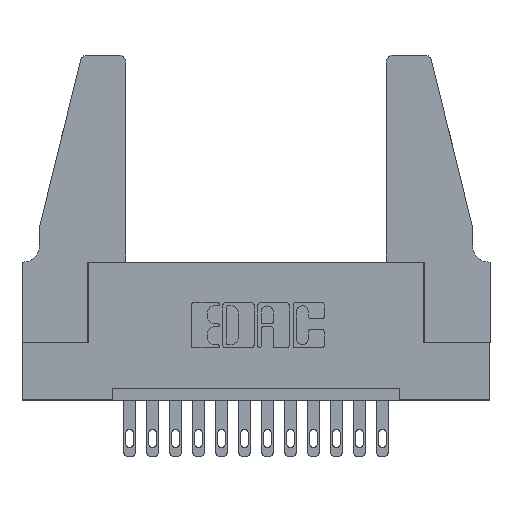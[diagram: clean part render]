
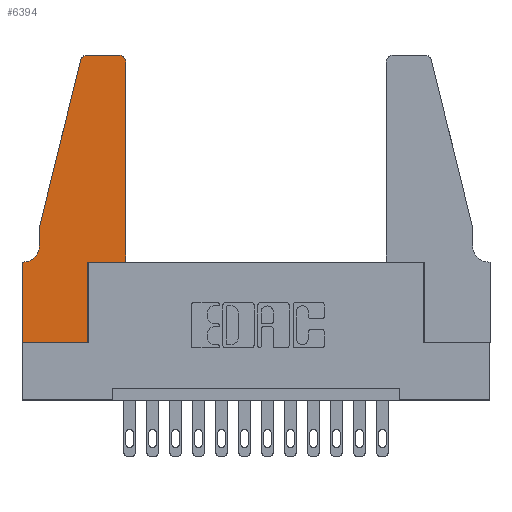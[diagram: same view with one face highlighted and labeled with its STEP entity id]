
A CAD part, top view. The second image highlights one B-rep face of the part: STEP entity #6394.
In plain terms, the highlighted planar face has unit normal (0, 0, 1).
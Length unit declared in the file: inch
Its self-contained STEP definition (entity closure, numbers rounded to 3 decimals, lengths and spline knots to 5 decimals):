
#30 = VERTEX_POINT ( 'NONE', #172 ) ;
#31 = CARTESIAN_POINT ( 'NONE',  ( 0.4505, 0.35, 0.37 ) ) ;
#32 = AXIS2_PLACEMENT_3D ( 'NONE', #9577, #11990, #8432 ) ;
#115 = CARTESIAN_POINT ( 'NONE',  ( 0.25487, 1.22718, 0.37 ) ) ;
#172 = CARTESIAN_POINT ( 'NONE',  ( 0.2865, 0.35, 0.37 ) ) ;
#289 = ORIENTED_EDGE ( 'NONE', *, *, #7589, .T. ) ;
#372 = ORIENTED_EDGE ( 'NONE', *, *, #15129, .T. ) ;
#528 = VECTOR ( 'NONE', #3207, 39.37008 ) ;
#712 = EDGE_CURVE ( 'NONE', #8361, #4221, #1528, .T. ) ;
#730 = CARTESIAN_POINT ( 'NONE',  ( 0.0055, 0.42, 0.37 ) ) ;
#919 = ORIENTED_EDGE ( 'NONE', *, *, #4706, .T. ) ;
#1107 = AXIS2_PLACEMENT_3D ( 'NONE', #2877, #8694, #6245 ) ;
#1387 = EDGE_CURVE ( 'NONE', #13014, #14418, #3705, .T. ) ;
#1528 = LINE ( 'NONE', #14785, #4673 ) ;
#1633 = EDGE_CURVE ( 'NONE', #4221, #30, #10145, .T. ) ;
#1637 = CARTESIAN_POINT ( 'NONE',  ( 0.4505, 1.22, 0.37 ) ) ;
#1676 = VECTOR ( 'NONE', #13841, 39.37008 ) ;
#1745 = CARTESIAN_POINT ( 'NONE',  ( 0., 0.35, 0.37 ) ) ;
#1811 = DIRECTION ( 'NONE',  ( 0., 0., 1. ) ) ;
#2015 = CARTESIAN_POINT ( 'NONE',  ( 0.0755, 0.5, 0.37 ) ) ;
#2060 = CARTESIAN_POINT ( 'NONE',  ( 0.284, 1.25, 0.37 ) ) ;
#2197 = LINE ( 'NONE', #2015, #528 ) ;
#2347 = LINE ( 'NONE', #13626, #3091 ) ;
#2384 = VERTEX_POINT ( 'NONE', #12942 ) ;
#2505 = DIRECTION ( 'NONE',  ( 1., 0., 0. ) ) ;
#2577 = CARTESIAN_POINT ( 'NONE',  ( 0.4505, 0.35, 0.37 ) ) ;
#2704 = LINE ( 'NONE', #10764, #11708 ) ;
#2785 = CIRCLE ( 'NONE', #12614, 0.07 ) ;
#2877 = CARTESIAN_POINT ( 'NONE',  ( 0.4205, 1.22, 0.37 ) ) ;
#3021 = DIRECTION ( 'NONE',  ( 1., 0., 0. ) ) ;
#3059 = PLANE ( 'NONE',  #10366 ) ;
#3091 = VECTOR ( 'NONE', #6474, 39.37008 ) ;
#3207 = DIRECTION ( 'NONE',  ( 0., -1., 0. ) ) ;
#3345 = EDGE_CURVE ( 'NONE', #12278, #14590, #2347, .T. ) ;
#3368 = VECTOR ( 'NONE', #6149, 39.37008 ) ;
#3610 = ORIENTED_EDGE ( 'NONE', *, *, #10073, .T. ) ;
#3705 = LINE ( 'NONE', #11720, #1676 ) ;
#4221 = VERTEX_POINT ( 'NONE', #15079 ) ;
#4346 = VERTEX_POINT ( 'NONE', #115 ) ;
#4609 = LINE ( 'NONE', #13821, #6424 ) ;
#4642 = CIRCLE ( 'NONE', #32, 0.03 ) ;
#4673 = VECTOR ( 'NONE', #6603, 39.37008 ) ;
#4704 = CIRCLE ( 'NONE', #1107, 0.03 ) ;
#4706 = EDGE_CURVE ( 'NONE', #14180, #12278, #4704, .T. ) ;
#5219 = ORIENTED_EDGE ( 'NONE', *, *, #13442, .T. ) ;
#5308 = ORIENTED_EDGE ( 'NONE', *, *, #712, .T. ) ;
#5489 = DIRECTION ( 'NONE',  ( -0.239, -0.971, 0. ) ) ;
#6100 = CARTESIAN_POINT ( 'NONE',  ( 0.2865, 0.35, 0.37 ) ) ;
#6149 = DIRECTION ( 'NONE',  ( 0., 1., 0. ) ) ;
#6245 = DIRECTION ( 'NONE',  ( 1., 0., 0. ) ) ;
#6394 = ADVANCED_FACE ( 'NONE', ( #14870 ), #3059, .T. ) ;
#6424 = VECTOR ( 'NONE', #5489, 39.37008 ) ;
#6474 = DIRECTION ( 'NONE',  ( -1., 0., 0. ) ) ;
#6603 = DIRECTION ( 'NONE',  ( 1., 0., 0. ) ) ;
#6948 = ORIENTED_EDGE ( 'NONE', *, *, #1387, .T. ) ;
#7041 = DIRECTION ( 'NONE',  ( 0., -1., 0. ) ) ;
#7384 = EDGE_CURVE ( 'NONE', #14590, #4346, #4642, .T. ) ;
#7427 = CARTESIAN_POINT ( 'NONE',  ( 0.4205, 1.25, 0.37 ) ) ;
#7589 = EDGE_CURVE ( 'NONE', #2384, #13014, #2785, .T. ) ;
#7730 = VECTOR ( 'NONE', #9360, 39.37008 ) ;
#8361 = VERTEX_POINT ( 'NONE', #8669 ) ;
#8432 = DIRECTION ( 'NONE',  ( 1., 0., 0. ) ) ;
#8627 = LINE ( 'NONE', #9400, #13401 ) ;
#8669 = CARTESIAN_POINT ( 'NONE',  ( 0., 0., 0.37 ) ) ;
#8694 = DIRECTION ( 'NONE',  ( 0., 0., 1. ) ) ;
#9360 = DIRECTION ( 'NONE',  ( 0., 1., 0. ) ) ;
#9400 = CARTESIAN_POINT ( 'NONE',  ( 0., 0., 0.37 ) ) ;
#9577 = CARTESIAN_POINT ( 'NONE',  ( 0.284, 1.22, 0.37 ) ) ;
#9772 = CARTESIAN_POINT ( 'NONE',  ( 0.0755, 0.5, 0.37 ) ) ;
#10073 = EDGE_CURVE ( 'NONE', #12759, #2384, #2197, .T. ) ;
#10145 = LINE ( 'NONE', #6100, #3368 ) ;
#10175 = ORIENTED_EDGE ( 'NONE', *, *, #11616, .T. ) ;
#10305 = ORIENTED_EDGE ( 'NONE', *, *, #7384, .T. ) ;
#10366 = AXIS2_PLACEMENT_3D ( 'NONE', #11344, #1811, #3021 ) ;
#10739 = CARTESIAN_POINT ( 'NONE',  ( 0.0055, 0.35, 0.37 ) ) ;
#10764 = CARTESIAN_POINT ( 'NONE',  ( 0.4505, 0.35, 0.37 ) ) ;
#11344 = CARTESIAN_POINT ( 'NONE',  ( 0., 0.35, 0.37 ) ) ;
#11354 = ORIENTED_EDGE ( 'NONE', *, *, #14095, .T. ) ;
#11616 = EDGE_CURVE ( 'NONE', #30, #12923, #2704, .T. ) ;
#11704 = ORIENTED_EDGE ( 'NONE', *, *, #1633, .T. ) ;
#11708 = VECTOR ( 'NONE', #2505, 39.37008 ) ;
#11720 = CARTESIAN_POINT ( 'NONE',  ( 0.0755, 0.35, 0.37 ) ) ;
#11990 = DIRECTION ( 'NONE',  ( 0., 0., 1. ) ) ;
#12212 = DIRECTION ( 'NONE',  ( 0., 0., -1. ) ) ;
#12278 = VERTEX_POINT ( 'NONE', #7427 ) ;
#12291 = EDGE_LOOP ( 'NONE', ( #13464, #10305, #372, #3610, #289, #6948, #11354, #5308, #11704, #10175, #5219, #919 ) ) ;
#12614 = AXIS2_PLACEMENT_3D ( 'NONE', #730, #12212, #15069 ) ;
#12759 = VERTEX_POINT ( 'NONE', #9772 ) ;
#12923 = VERTEX_POINT ( 'NONE', #2577 ) ;
#12942 = CARTESIAN_POINT ( 'NONE',  ( 0.0755, 0.42, 0.37 ) ) ;
#13014 = VERTEX_POINT ( 'NONE', #10739 ) ;
#13401 = VECTOR ( 'NONE', #7041, 39.37008 ) ;
#13442 = EDGE_CURVE ( 'NONE', #12923, #14180, #14516, .T. ) ;
#13464 = ORIENTED_EDGE ( 'NONE', *, *, #3345, .T. ) ;
#13626 = CARTESIAN_POINT ( 'NONE',  ( 0.2605, 1.25, 0.37 ) ) ;
#13821 = CARTESIAN_POINT ( 'NONE',  ( 0.0755, 0.5, 0.37 ) ) ;
#13841 = DIRECTION ( 'NONE',  ( -1., 0., 0. ) ) ;
#14095 = EDGE_CURVE ( 'NONE', #14418, #8361, #8627, .T. ) ;
#14180 = VERTEX_POINT ( 'NONE', #1637 ) ;
#14418 = VERTEX_POINT ( 'NONE', #1745 ) ;
#14516 = LINE ( 'NONE', #31, #7730 ) ;
#14590 = VERTEX_POINT ( 'NONE', #2060 ) ;
#14785 = CARTESIAN_POINT ( 'NONE',  ( 0., 0., 0.37 ) ) ;
#14870 = FACE_OUTER_BOUND ( 'NONE', #12291, .T. ) ;
#15069 = DIRECTION ( 'NONE',  ( -1., 0., 0. ) ) ;
#15079 = CARTESIAN_POINT ( 'NONE',  ( 0.2865, 0., 0.37 ) ) ;
#15129 = EDGE_CURVE ( 'NONE', #4346, #12759, #4609, .T. ) ;
